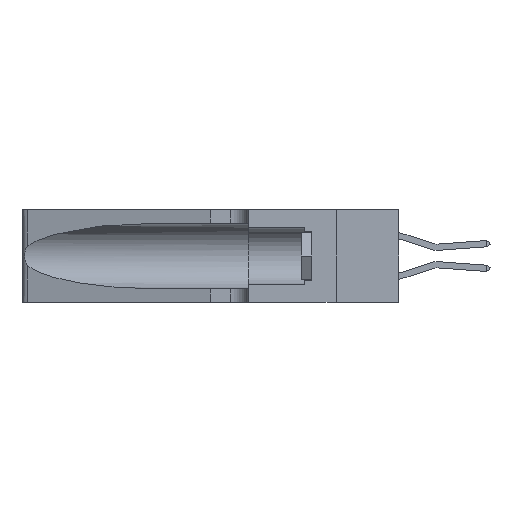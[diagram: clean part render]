
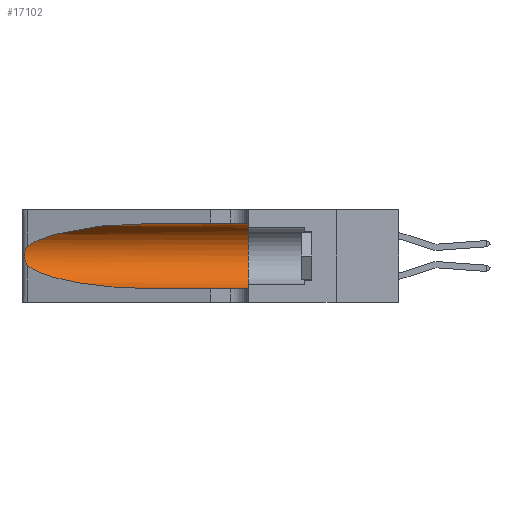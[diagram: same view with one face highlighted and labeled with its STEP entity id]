
A CAD part, left-side view. The second image highlights one B-rep face of the part: STEP entity #17102.
In plain terms, the highlighted cylindrical face has radius 3.308 mm (diameter 6.617 mm), a partial arc.
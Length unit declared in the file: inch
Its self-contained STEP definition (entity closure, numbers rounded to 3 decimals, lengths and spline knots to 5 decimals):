
#32 = AXIS2_PLACEMENT_3D ( 'NONE', #23246, #7812, #700 ) ;
#123 = B_SPLINE_CURVE_WITH_KNOTS ( 'NONE', 3,
 ( #8750, #15568, #8352, #22428, #13212, #17972, #17871, #22333, #29217, #11078, #3670, #3979, #10784, #15670 ),
 .UNSPECIFIED., .F., .F.,
 ( 4, 2, 2, 2, 2, 2, 4 ),
 ( 0., 0.00027, 0.00053, 0.00107, 0.0016, 0.00187, 0.00214 ),
 .UNSPECIFIED. ) ;
#288 = CARTESIAN_POINT ( 'NONE',  ( 0.25487, 1.22718, 0.14631 ) ) ;
#700 = DIRECTION ( 'NONE',  ( 0., 0., -1. ) ) ;
#843 = EDGE_CURVE ( 'NONE', #21543, #4754, #5148, .T. ) ;
#1141 = CARTESIAN_POINT ( 'NONE',  ( 0.2373, 1.15595, 0.28018 ) ) ;
#1942 = ORIENTED_EDGE ( 'NONE', *, *, #21035, .T. ) ;
#3265 = ORIENTED_EDGE ( 'NONE', *, *, #14039, .T. ) ;
#3617 = EDGE_CURVE ( 'NONE', #27598, #25428, #12370, .T. ) ;
#3670 = CARTESIAN_POINT ( 'NONE',  ( 0.25789, 1.23486, 0.15765 ) ) ;
#3819 = CARTESIAN_POINT ( 'NONE',  ( 0.18966, 0.96281, 0.05475 ) ) ;
#3979 = CARTESIAN_POINT ( 'NONE',  ( 0.25639, 1.23186, 0.15144 ) ) ;
#4754 = VERTEX_POINT ( 'NONE', #22046 ) ;
#5148 =( BOUNDED_CURVE ( )  B_SPLINE_CURVE ( 3, ( #28956, #10820, #3819, #13154 ),
 .UNSPECIFIED., .F., .F. ) 
 B_SPLINE_CURVE_WITH_KNOTS ( ( 4, 4 ),
 ( 3.44316, 4.71239 ),
 .UNSPECIFIED. ) 
 CURVE ( )  GEOMETRIC_REPRESENTATION_ITEM ( )  RATIONAL_B_SPLINE_CURVE ( ( 1., 0.87, 0.87, 1. ) ) 
 REPRESENTATION_ITEM ( '' )  );
#5521 = EDGE_CURVE ( 'NONE', #24998, #27598, #18427, .T. ) ;
#5719 = CARTESIAN_POINT ( 'NONE',  ( 0.1305, 1.61858, 0.31525 ) ) ;
#7619 = ORIENTED_EDGE ( 'NONE', *, *, #17493, .T. ) ;
#7735 = DIRECTION ( 'NONE',  ( 0., 1., 0. ) ) ;
#7812 = DIRECTION ( 'NONE',  ( 0., -1., 0. ) ) ;
#8056 = CARTESIAN_POINT ( 'NONE',  ( 0.1305, 0.72297, 0.31525 ) ) ;
#8352 = CARTESIAN_POINT ( 'NONE',  ( 0.25639, 1.23184, 0.21858 ) ) ;
#8359 = CARTESIAN_POINT ( 'NONE',  ( 0.25487, 1.22718, 0.22369 ) ) ;
#8750 = CARTESIAN_POINT ( 'NONE',  ( 0.25487, 1.22718, 0.22369 ) ) ;
#9536 = VERTEX_POINT ( 'NONE', #11665 ) ;
#10784 = CARTESIAN_POINT ( 'NONE',  ( 0.25555, 1.22993, 0.14849 ) ) ;
#10820 = CARTESIAN_POINT ( 'NONE',  ( 0.2373, 1.15595, 0.08982 ) ) ;
#11078 = CARTESIAN_POINT ( 'NONE',  ( 0.25856, 1.23593, 0.16098 ) ) ;
#11573 = CARTESIAN_POINT ( 'NONE',  ( 0.1305, 0.72297, 0.31525 ) ) ;
#11665 = CARTESIAN_POINT ( 'NONE',  ( 0.25487, 1.22718, 0.22369 ) ) ;
#12109 = CYLINDRICAL_SURFACE ( 'NONE', #32, 0.13025 ) ;
#12369 = CARTESIAN_POINT ( 'NONE',  ( 0.1305, 0.35, 0.31525 ) ) ;
#12370 = CIRCLE ( 'NONE', #13234, 0.13025 ) ;
#13154 = CARTESIAN_POINT ( 'NONE',  ( 0.1305, 0.72297, 0.05475 ) ) ;
#13212 = CARTESIAN_POINT ( 'NONE',  ( 0.25854, 1.2359, 0.20912 ) ) ;
#13234 = AXIS2_PLACEMENT_3D ( 'NONE', #23856, #7735, #23953 ) ;
#14039 = EDGE_CURVE ( 'NONE', #9536, #21543, #123, .T. ) ;
#14093 =( BOUNDED_CURVE ( )  B_SPLINE_CURVE ( 3, ( #8056, #26844, #1141, #8359 ),
 .UNSPECIFIED., .F., .T. ) 
 B_SPLINE_CURVE_WITH_KNOTS ( ( 4, 4 ),
 ( 1.5708, 2.84003 ),
 .UNSPECIFIED. ) 
 CURVE ( )  GEOMETRIC_REPRESENTATION_ITEM ( )  RATIONAL_B_SPLINE_CURVE ( ( 1., 0.87, 0.87, 1. ) ) 
 REPRESENTATION_ITEM ( '' )  );
#15133 = ORIENTED_EDGE ( 'NONE', *, *, #5521, .F. ) ;
#15291 = EDGE_LOOP ( 'NONE', ( #1942, #3265, #17989, #7619, #26855, #15133 ) ) ;
#15568 = CARTESIAN_POINT ( 'NONE',  ( 0.25555, 1.22994, 0.2215 ) ) ;
#15670 = CARTESIAN_POINT ( 'NONE',  ( 0.25487, 1.22718, 0.14631 ) ) ;
#16090 = FACE_OUTER_BOUND ( 'NONE', #15291, .T. ) ;
#16545 = CARTESIAN_POINT ( 'NONE',  ( 0.1305, 0.35, 0.05475 ) ) ;
#17102 = ADVANCED_FACE ( 'NONE', ( #16090 ), #12109, .F. ) ;
#17493 = EDGE_CURVE ( 'NONE', #4754, #25428, #19686, .T. ) ;
#17871 = CARTESIAN_POINT ( 'NONE',  ( 0.26075, 1.23896, 0.19203 ) ) ;
#17972 = CARTESIAN_POINT ( 'NONE',  ( 0.26018, 1.23835, 0.19895 ) ) ;
#17989 = ORIENTED_EDGE ( 'NONE', *, *, #843, .T. ) ;
#18427 = LINE ( 'NONE', #5719, #22380 ) ;
#19686 = LINE ( 'NONE', #23515, #24032 ) ;
#21035 = EDGE_CURVE ( 'NONE', #24998, #9536, #14093, .T. ) ;
#21543 = VERTEX_POINT ( 'NONE', #288 ) ;
#22046 = CARTESIAN_POINT ( 'NONE',  ( 0.1305, 0.72297, 0.05475 ) ) ;
#22333 = CARTESIAN_POINT ( 'NONE',  ( 0.26075, 1.23896, 0.178 ) ) ;
#22380 = VECTOR ( 'NONE', #22429, 39.37008 ) ;
#22428 = CARTESIAN_POINT ( 'NONE',  ( 0.25787, 1.23484, 0.2124 ) ) ;
#22429 = DIRECTION ( 'NONE',  ( 0., -1., 0. ) ) ;
#23246 = CARTESIAN_POINT ( 'NONE',  ( 0.1305, 1.61858, 0.185 ) ) ;
#23515 = CARTESIAN_POINT ( 'NONE',  ( 0.1305, 1.61858, 0.05475 ) ) ;
#23856 = CARTESIAN_POINT ( 'NONE',  ( 0.1305, 0.35, 0.185 ) ) ;
#23953 = DIRECTION ( 'NONE',  ( 0., 0., 1. ) ) ;
#24032 = VECTOR ( 'NONE', #27997, 39.37008 ) ;
#24998 = VERTEX_POINT ( 'NONE', #11573 ) ;
#25428 = VERTEX_POINT ( 'NONE', #16545 ) ;
#26844 = CARTESIAN_POINT ( 'NONE',  ( 0.18966, 0.96281, 0.31525 ) ) ;
#26855 = ORIENTED_EDGE ( 'NONE', *, *, #3617, .F. ) ;
#27598 = VERTEX_POINT ( 'NONE', #12369 ) ;
#27997 = DIRECTION ( 'NONE',  ( 0., -1., 0. ) ) ;
#28956 = CARTESIAN_POINT ( 'NONE',  ( 0.25487, 1.22718, 0.14631 ) ) ;
#29217 = CARTESIAN_POINT ( 'NONE',  ( 0.26017, 1.23833, 0.17102 ) ) ;
